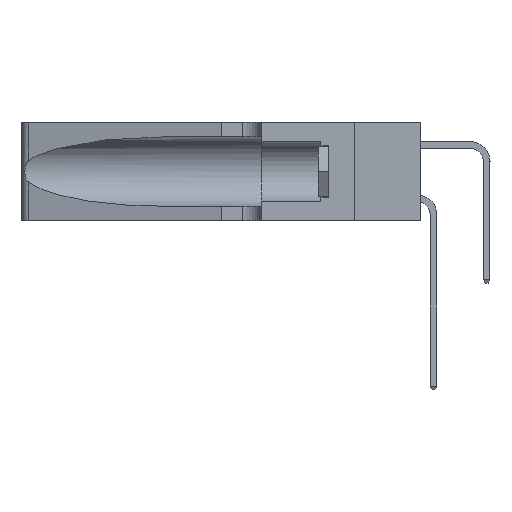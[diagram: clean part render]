
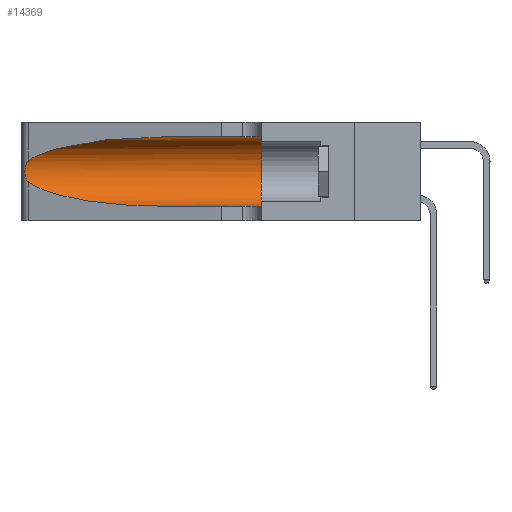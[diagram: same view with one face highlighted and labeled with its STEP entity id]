
A CAD part, left-side view. The second image highlights one B-rep face of the part: STEP entity #14369.
In plain terms, the highlighted cylindrical face has radius 3.308 mm (diameter 6.617 mm), a partial arc.
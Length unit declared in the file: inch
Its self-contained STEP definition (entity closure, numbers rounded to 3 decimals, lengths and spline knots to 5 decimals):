
#87 = CARTESIAN_POINT ( 'NONE',  ( 0.1305, 0.72297, 0.31525 ) ) ;
#210 = LINE ( 'NONE', #12503, #10112 ) ;
#426 = ORIENTED_EDGE ( 'NONE', *, *, #18554, .F. ) ;
#451 = ORIENTED_EDGE ( 'NONE', *, *, #12567, .T. ) ;
#693 = CARTESIAN_POINT ( 'NONE',  ( 0.25487, 1.22718, 0.14631 ) ) ;
#826 = CARTESIAN_POINT ( 'NONE',  ( 0.26018, 1.23835, 0.19895 ) ) ;
#1468 = EDGE_CURVE ( 'NONE', #18598, #9049, #16868, .T. ) ;
#2172 = FACE_OUTER_BOUND ( 'NONE', #15646, .T. ) ;
#2227 = CARTESIAN_POINT ( 'NONE',  ( 0.26075, 1.23896, 0.178 ) ) ;
#2574 = ORIENTED_EDGE ( 'NONE', *, *, #1468, .T. ) ;
#3228 = CARTESIAN_POINT ( 'NONE',  ( 0.1305, 0.72297, 0.05475 ) ) ;
#3419 = EDGE_CURVE ( 'NONE', #9624, #18598, #16421, .T. ) ;
#3674 = ORIENTED_EDGE ( 'NONE', *, *, #15833, .F. ) ;
#3802 = CARTESIAN_POINT ( 'NONE',  ( 0.2373, 1.15595, 0.08982 ) ) ;
#4281 = VERTEX_POINT ( 'NONE', #10992 ) ;
#5461 = CARTESIAN_POINT ( 'NONE',  ( 0.26075, 1.23896, 0.19203 ) ) ;
#5529 = CARTESIAN_POINT ( 'NONE',  ( 0.1305, 0.72297, 0.31525 ) ) ;
#5725 = CARTESIAN_POINT ( 'NONE',  ( 0.1305, 1.61858, 0.185 ) ) ;
#6995 = CARTESIAN_POINT ( 'NONE',  ( 0.1305, 0.35, 0.31525 ) ) ;
#7093 = CARTESIAN_POINT ( 'NONE',  ( 0.18966, 0.96281, 0.31525 ) ) ;
#7156 = VERTEX_POINT ( 'NONE', #87 ) ;
#8165 = CARTESIAN_POINT ( 'NONE',  ( 0.1305, 0.35, 0.05475 ) ) ;
#8509 = CARTESIAN_POINT ( 'NONE',  ( 0.25787, 1.23484, 0.2124 ) ) ;
#8754 = CARTESIAN_POINT ( 'NONE',  ( 0.25487, 1.22718, 0.14631 ) ) ;
#9049 = VERTEX_POINT ( 'NONE', #8165 ) ;
#9109 = DIRECTION ( 'NONE',  ( 0., -1., 0. ) ) ;
#9542 = DIRECTION ( 'NONE',  ( 0., 0., 1. ) ) ;
#9624 = VERTEX_POINT ( 'NONE', #10809 ) ;
#9917 = B_SPLINE_CURVE_WITH_KNOTS ( 'NONE', 3,
 ( #14616, #9941, #11691, #8509, #13081, #826, #5461, #2227, #19032, #11553, #12893, #16227, #19299, #693 ),
 .UNSPECIFIED., .F., .F.,
 ( 4, 2, 2, 2, 2, 2, 4 ),
 ( 0., 0.00027, 0.00053, 0.00107, 0.0016, 0.00187, 0.00214 ),
 .UNSPECIFIED. ) ;
#9941 = CARTESIAN_POINT ( 'NONE',  ( 0.25555, 1.22994, 0.2215 ) ) ;
#10112 = VECTOR ( 'NONE', #12434, 39.37008 ) ;
#10809 = CARTESIAN_POINT ( 'NONE',  ( 0.25487, 1.22718, 0.14631 ) ) ;
#10992 = CARTESIAN_POINT ( 'NONE',  ( 0.25487, 1.22718, 0.22369 ) ) ;
#11553 = CARTESIAN_POINT ( 'NONE',  ( 0.25856, 1.23593, 0.16098 ) ) ;
#11617 = CYLINDRICAL_SURFACE ( 'NONE', #15874, 0.13025 ) ;
#11662 = CARTESIAN_POINT ( 'NONE',  ( 0.18966, 0.96281, 0.05475 ) ) ;
#11691 = CARTESIAN_POINT ( 'NONE',  ( 0.25639, 1.23184, 0.21858 ) ) ;
#12150 = DIRECTION ( 'NONE',  ( 0., 0., -1. ) ) ;
#12250 =( BOUNDED_CURVE ( )  B_SPLINE_CURVE ( 3, ( #5529, #7093, #14872, #13274 ),
 .UNSPECIFIED., .F., .F. ) 
 B_SPLINE_CURVE_WITH_KNOTS ( ( 4, 4 ),
 ( 1.5708, 2.84003 ),
 .UNSPECIFIED. ) 
 CURVE ( )  GEOMETRIC_REPRESENTATION_ITEM ( )  RATIONAL_B_SPLINE_CURVE ( ( 1., 0.87, 0.87, 1. ) ) 
 REPRESENTATION_ITEM ( '' )  );
#12321 = EDGE_CURVE ( 'NONE', #4281, #9624, #9917, .T. ) ;
#12434 = DIRECTION ( 'NONE',  ( 0., -1., 0. ) ) ;
#12503 = CARTESIAN_POINT ( 'NONE',  ( 0.1305, 1.61858, 0.31525 ) ) ;
#12567 = EDGE_CURVE ( 'NONE', #7156, #4281, #12250, .T. ) ;
#12893 = CARTESIAN_POINT ( 'NONE',  ( 0.25789, 1.23486, 0.15765 ) ) ;
#13081 = CARTESIAN_POINT ( 'NONE',  ( 0.25854, 1.2359, 0.20912 ) ) ;
#13274 = CARTESIAN_POINT ( 'NONE',  ( 0.25487, 1.22718, 0.22369 ) ) ;
#14369 = ADVANCED_FACE ( 'NONE', ( #2172 ), #11617, .F. ) ;
#14423 = CARTESIAN_POINT ( 'NONE',  ( 0.1305, 1.61858, 0.05475 ) ) ;
#14616 = CARTESIAN_POINT ( 'NONE',  ( 0.25487, 1.22718, 0.22369 ) ) ;
#14872 = CARTESIAN_POINT ( 'NONE',  ( 0.2373, 1.15595, 0.28018 ) ) ;
#14983 = AXIS2_PLACEMENT_3D ( 'NONE', #15627, #18714, #9542 ) ;
#15627 = CARTESIAN_POINT ( 'NONE',  ( 0.1305, 0.35, 0.185 ) ) ;
#15646 = EDGE_LOOP ( 'NONE', ( #451, #19654, #17655, #2574, #3674, #426 ) ) ;
#15833 = EDGE_CURVE ( 'NONE', #19309, #9049, #19434, .T. ) ;
#15874 = AXIS2_PLACEMENT_3D ( 'NONE', #5725, #9109, #12150 ) ;
#16227 = CARTESIAN_POINT ( 'NONE',  ( 0.25639, 1.23186, 0.15144 ) ) ;
#16421 =( BOUNDED_CURVE ( )  B_SPLINE_CURVE ( 3, ( #8754, #3802, #11662, #17673 ),
 .UNSPECIFIED., .F., .F. ) 
 B_SPLINE_CURVE_WITH_KNOTS ( ( 4, 4 ),
 ( 3.44316, 4.71239 ),
 .UNSPECIFIED. ) 
 CURVE ( )  GEOMETRIC_REPRESENTATION_ITEM ( )  RATIONAL_B_SPLINE_CURVE ( ( 1., 0.87, 0.87, 1. ) ) 
 REPRESENTATION_ITEM ( '' )  );
#16868 = LINE ( 'NONE', #14423, #19487 ) ;
#17655 = ORIENTED_EDGE ( 'NONE', *, *, #3419, .T. ) ;
#17673 = CARTESIAN_POINT ( 'NONE',  ( 0.1305, 0.72297, 0.05475 ) ) ;
#18554 = EDGE_CURVE ( 'NONE', #7156, #19309, #210, .T. ) ;
#18598 = VERTEX_POINT ( 'NONE', #3228 ) ;
#18714 = DIRECTION ( 'NONE',  ( 0., 1., 0. ) ) ;
#19032 = CARTESIAN_POINT ( 'NONE',  ( 0.26017, 1.23833, 0.17102 ) ) ;
#19187 = DIRECTION ( 'NONE',  ( 0., -1., 0. ) ) ;
#19299 = CARTESIAN_POINT ( 'NONE',  ( 0.25555, 1.22993, 0.14849 ) ) ;
#19309 = VERTEX_POINT ( 'NONE', #6995 ) ;
#19434 = CIRCLE ( 'NONE', #14983, 0.13025 ) ;
#19487 = VECTOR ( 'NONE', #19187, 39.37008 ) ;
#19654 = ORIENTED_EDGE ( 'NONE', *, *, #12321, .T. ) ;
